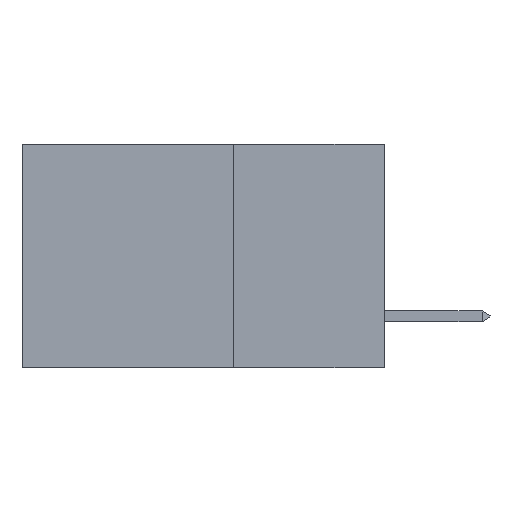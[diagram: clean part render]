
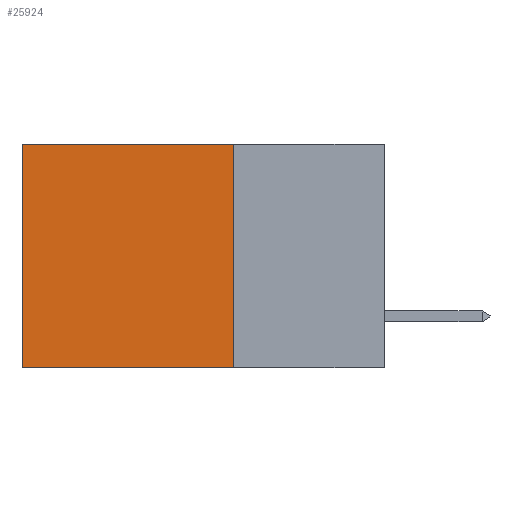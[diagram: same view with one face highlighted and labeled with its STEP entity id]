
A CAD part, left-side view. The second image highlights one B-rep face of the part: STEP entity #25924.
In plain terms, the highlighted planar face has unit normal (-1, 0, 0).
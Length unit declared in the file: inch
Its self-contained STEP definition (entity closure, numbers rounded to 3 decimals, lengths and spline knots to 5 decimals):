
#1173 = CARTESIAN_POINT ( 'NONE',  ( 0.2875, 0.25, 0. ) ) ;
#1209 = VERTEX_POINT ( 'NONE', #19901 ) ;
#2688 = DIRECTION ( 'NONE',  ( 0., 1., 0. ) ) ;
#3124 = CARTESIAN_POINT ( 'NONE',  ( 0.2875, 0.25, 0. ) ) ;
#4691 = VECTOR ( 'NONE', #31391, 39.37008 ) ;
#4867 = LINE ( 'NONE', #23256, #14600 ) ;
#5054 = VERTEX_POINT ( 'NONE', #22045 ) ;
#7645 = EDGE_LOOP ( 'NONE', ( #11710, #32219, #13419, #30809 ) ) ;
#8846 = EDGE_CURVE ( 'NONE', #16091, #5054, #16115, .T. ) ;
#10025 = AXIS2_PLACEMENT_3D ( 'NONE', #3124, #18215, #24807 ) ;
#11242 = VERTEX_POINT ( 'NONE', #1173 ) ;
#11710 = ORIENTED_EDGE ( 'NONE', *, *, #8846, .T. ) ;
#12017 = FACE_OUTER_BOUND ( 'NONE', #7645, .T. ) ;
#13419 = ORIENTED_EDGE ( 'NONE', *, *, #21172, .F. ) ;
#14600 = VECTOR ( 'NONE', #20563, 39.37008 ) ;
#15586 = EDGE_CURVE ( 'NONE', #1209, #5054, #30564, .T. ) ;
#16091 = VERTEX_POINT ( 'NONE', #37123 ) ;
#16115 = LINE ( 'NONE', #18808, #4691 ) ;
#16614 = DIRECTION ( 'NONE',  ( 0., 1., 0. ) ) ;
#18215 = DIRECTION ( 'NONE',  ( 1., 0., 0. ) ) ;
#18808 = CARTESIAN_POINT ( 'NONE',  ( 0.2875, 0.6, 0. ) ) ;
#19901 = CARTESIAN_POINT ( 'NONE',  ( 0.2875, 0.25, -0.37 ) ) ;
#20116 = LINE ( 'NONE', #32089, #37184 ) ;
#20563 = DIRECTION ( 'NONE',  ( 0., 0., -1. ) ) ;
#21172 = EDGE_CURVE ( 'NONE', #11242, #1209, #4867, .T. ) ;
#22045 = CARTESIAN_POINT ( 'NONE',  ( 0.2875, 0.6, -0.37 ) ) ;
#23256 = CARTESIAN_POINT ( 'NONE',  ( 0.2875, 0.25, 0. ) ) ;
#24807 = DIRECTION ( 'NONE',  ( 0., 0., -1. ) ) ;
#25924 = ADVANCED_FACE ( 'NONE', ( #12017 ), #34509, .F. ) ;
#30564 = LINE ( 'NONE', #37167, #33951 ) ;
#30809 = ORIENTED_EDGE ( 'NONE', *, *, #31048, .T. ) ;
#31048 = EDGE_CURVE ( 'NONE', #11242, #16091, #20116, .T. ) ;
#31391 = DIRECTION ( 'NONE',  ( 0., 0., -1. ) ) ;
#32089 = CARTESIAN_POINT ( 'NONE',  ( 0.2875, 0.25, 0. ) ) ;
#32219 = ORIENTED_EDGE ( 'NONE', *, *, #15586, .F. ) ;
#33951 = VECTOR ( 'NONE', #2688, 39.37008 ) ;
#34509 = PLANE ( 'NONE',  #10025 ) ;
#37123 = CARTESIAN_POINT ( 'NONE',  ( 0.2875, 0.6, 0. ) ) ;
#37167 = CARTESIAN_POINT ( 'NONE',  ( 0.2875, 0.25, -0.37 ) ) ;
#37184 = VECTOR ( 'NONE', #16614, 39.37008 ) ;
